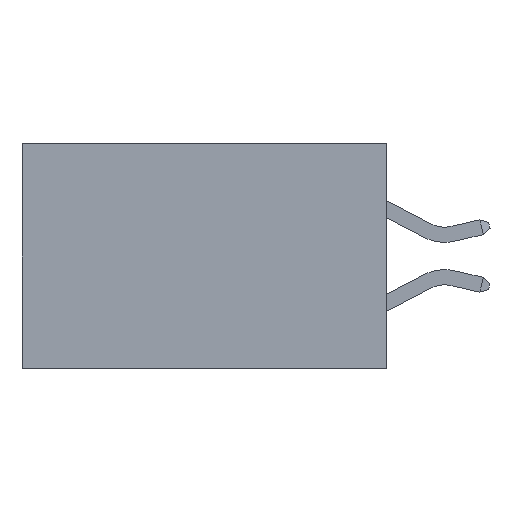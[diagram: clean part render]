
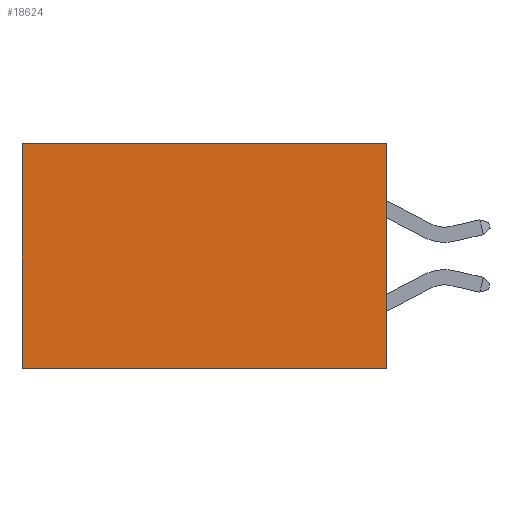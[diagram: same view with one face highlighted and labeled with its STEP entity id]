
A CAD part, left-side view. The second image highlights one B-rep face of the part: STEP entity #18624.
In plain terms, the highlighted planar face has unit normal (-1, 0, 0).
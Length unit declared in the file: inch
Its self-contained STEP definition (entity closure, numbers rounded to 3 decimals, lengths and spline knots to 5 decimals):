
#1403 = DIRECTION ( 'NONE',  ( 1., 0., 0. ) ) ;
#3487 = ORIENTED_EDGE ( 'NONE', *, *, #5820, .F. ) ;
#4022 = CARTESIAN_POINT ( 'NONE',  ( 0.2615, 0., -0.37 ) ) ;
#4080 = LINE ( 'NONE', #15556, #14371 ) ;
#4135 = DIRECTION ( 'NONE',  ( 0., 1., 0. ) ) ;
#4576 = CARTESIAN_POINT ( 'NONE',  ( 0.2615, 0., -0.37 ) ) ;
#5255 = DIRECTION ( 'NONE',  ( 0., 0., -1. ) ) ;
#5820 = EDGE_CURVE ( 'NONE', #16259, #11858, #18454, .T. ) ;
#6166 = PLANE ( 'NONE',  #20515 ) ;
#7238 = VECTOR ( 'NONE', #4135, 39.37008 ) ;
#7379 = CARTESIAN_POINT ( 'NONE',  ( 0.2615, 0., 0. ) ) ;
#9180 = VERTEX_POINT ( 'NONE', #12620 ) ;
#9215 = DIRECTION ( 'NONE',  ( 0., 0., -1. ) ) ;
#10089 = LINE ( 'NONE', #16409, #14060 ) ;
#10496 = DIRECTION ( 'NONE',  ( 0., 1., 0. ) ) ;
#11145 = EDGE_CURVE ( 'NONE', #16259, #14283, #4080, .T. ) ;
#11858 = VERTEX_POINT ( 'NONE', #16037 ) ;
#12013 = DIRECTION ( 'NONE',  ( 0., 0., -1. ) ) ;
#12236 = CARTESIAN_POINT ( 'NONE',  ( 0.2615, 0., -0.37 ) ) ;
#12620 = CARTESIAN_POINT ( 'NONE',  ( 0.2615, 0.6, -0.37 ) ) ;
#13322 = EDGE_CURVE ( 'NONE', #11858, #9180, #18574, .T. ) ;
#13638 = EDGE_LOOP ( 'NONE', ( #20124, #16841, #3487, #14810 ) ) ;
#14060 = VECTOR ( 'NONE', #5255, 39.37008 ) ;
#14283 = VERTEX_POINT ( 'NONE', #15248 ) ;
#14371 = VECTOR ( 'NONE', #10496, 39.37008 ) ;
#14810 = ORIENTED_EDGE ( 'NONE', *, *, #11145, .T. ) ;
#15248 = CARTESIAN_POINT ( 'NONE',  ( 0.2615, 0.6, 0. ) ) ;
#15556 = CARTESIAN_POINT ( 'NONE',  ( 0.2615, 0., 0. ) ) ;
#15832 = FACE_OUTER_BOUND ( 'NONE', #13638, .T. ) ;
#16037 = CARTESIAN_POINT ( 'NONE',  ( 0.2615, 0., -0.37 ) ) ;
#16259 = VERTEX_POINT ( 'NONE', #7379 ) ;
#16409 = CARTESIAN_POINT ( 'NONE',  ( 0.2615, 0.6, -0.37 ) ) ;
#16568 = EDGE_CURVE ( 'NONE', #14283, #9180, #10089, .T. ) ;
#16841 = ORIENTED_EDGE ( 'NONE', *, *, #13322, .F. ) ;
#18227 = VECTOR ( 'NONE', #12013, 39.37008 ) ;
#18454 = LINE ( 'NONE', #4022, #18227 ) ;
#18574 = LINE ( 'NONE', #12236, #7238 ) ;
#18624 = ADVANCED_FACE ( 'NONE', ( #15832 ), #6166, .F. ) ;
#20124 = ORIENTED_EDGE ( 'NONE', *, *, #16568, .T. ) ;
#20515 = AXIS2_PLACEMENT_3D ( 'NONE', #4576, #1403, #9215 ) ;
